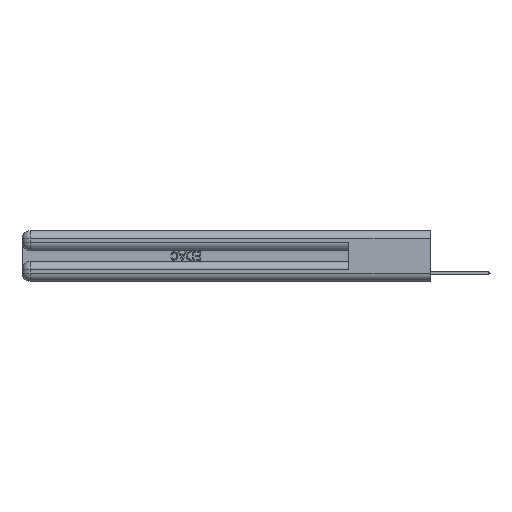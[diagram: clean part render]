
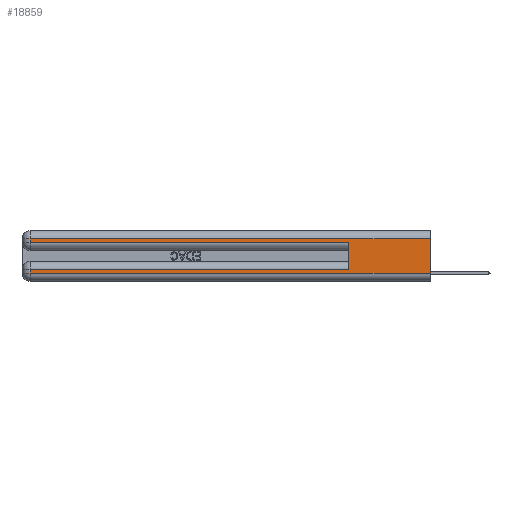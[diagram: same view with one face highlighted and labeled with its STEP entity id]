
A CAD part, left-side view. The second image highlights one B-rep face of the part: STEP entity #18859.
In plain terms, the highlighted planar face has unit normal (-1, 0, 0).
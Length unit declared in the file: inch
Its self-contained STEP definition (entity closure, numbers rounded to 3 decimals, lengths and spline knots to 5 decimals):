
#76 = CARTESIAN_POINT ( 'NONE',  ( 0., 2.94, 0.285 ) ) ;
#77 = DIRECTION ( 'NONE',  ( 0., 1., 0. ) ) ;
#915 = VERTEX_POINT ( 'NONE', #26305 ) ;
#960 = CARTESIAN_POINT ( 'NONE',  ( 0., 2.94, 0.085 ) ) ;
#1370 = DIRECTION ( 'NONE',  ( 0., 1., 0. ) ) ;
#1757 = CARTESIAN_POINT ( 'NONE',  ( 0., 0., 0.085 ) ) ;
#2196 = LINE ( 'NONE', #12408, #24344 ) ;
#2797 = VECTOR ( 'NONE', #77, 39.37008 ) ;
#3200 = VERTEX_POINT ( 'NONE', #20789 ) ;
#4183 = DIRECTION ( 'NONE',  ( 0., 0., -1. ) ) ;
#4246 = LINE ( 'NONE', #13403, #15319 ) ;
#4471 = VECTOR ( 'NONE', #8225, 39.37008 ) ;
#4505 = EDGE_CURVE ( 'NONE', #9222, #26386, #4246, .T. ) ;
#4554 = VECTOR ( 'NONE', #13095, 39.37008 ) ;
#5311 = EDGE_CURVE ( 'NONE', #12001, #16558, #11518, .T. ) ;
#6048 = AXIS2_PLACEMENT_3D ( 'NONE', #17595, #20907, #12003 ) ;
#7359 = ORIENTED_EDGE ( 'NONE', *, *, #26562, .T. ) ;
#8225 = DIRECTION ( 'NONE',  ( 0., 0., -1. ) ) ;
#8251 = CARTESIAN_POINT ( 'NONE',  ( 0., 2.94, 0.37 ) ) ;
#9196 = ORIENTED_EDGE ( 'NONE', *, *, #4505, .F. ) ;
#9222 = VERTEX_POINT ( 'NONE', #20706 ) ;
#9825 = ORIENTED_EDGE ( 'NONE', *, *, #13390, .F. ) ;
#10699 = CARTESIAN_POINT ( 'NONE',  ( 0., 0., 0.285 ) ) ;
#11518 = LINE ( 'NONE', #1757, #2797 ) ;
#12001 = VERTEX_POINT ( 'NONE', #29136 ) ;
#12003 = DIRECTION ( 'NONE',  ( 0., 0., -1. ) ) ;
#12088 = ORIENTED_EDGE ( 'NONE', *, *, #16256, .T. ) ;
#12408 = CARTESIAN_POINT ( 'NONE',  ( 0., 0., 0.06 ) ) ;
#12576 = VERTEX_POINT ( 'NONE', #21124 ) ;
#13095 = DIRECTION ( 'NONE',  ( 0., -1., 0. ) ) ;
#13332 = LINE ( 'NONE', #8251, #26271 ) ;
#13390 = EDGE_CURVE ( 'NONE', #12001, #12576, #27949, .T. ) ;
#13403 = CARTESIAN_POINT ( 'NONE',  ( 0., 0., 0.37 ) ) ;
#14006 = ORIENTED_EDGE ( 'NONE', *, *, #20145, .T. ) ;
#14371 = DIRECTION ( 'NONE',  ( 0., -1., 0. ) ) ;
#14449 = EDGE_CURVE ( 'NONE', #16558, #915, #13332, .T. ) ;
#14635 = EDGE_CURVE ( 'NONE', #915, #26386, #2196, .T. ) ;
#15008 = ORIENTED_EDGE ( 'NONE', *, *, #14635, .T. ) ;
#15319 = VECTOR ( 'NONE', #22906, 39.37008 ) ;
#15427 = CARTESIAN_POINT ( 'NONE',  ( 0., 0., 0.06 ) ) ;
#16256 = EDGE_CURVE ( 'NONE', #3200, #17463, #19938, .T. ) ;
#16558 = VERTEX_POINT ( 'NONE', #960 ) ;
#17441 = ORIENTED_EDGE ( 'NONE', *, *, #5311, .T. ) ;
#17463 = VERTEX_POINT ( 'NONE', #76 ) ;
#17465 = LINE ( 'NONE', #19732, #19450 ) ;
#17595 = CARTESIAN_POINT ( 'NONE',  ( 0., 0., 0.37 ) ) ;
#17645 = LINE ( 'NONE', #10699, #4554 ) ;
#18859 = ADVANCED_FACE ( 'NONE', ( #24674 ), #22419, .F. ) ;
#19450 = VECTOR ( 'NONE', #1370, 39.37008 ) ;
#19626 = VECTOR ( 'NONE', #25542, 39.37008 ) ;
#19732 = CARTESIAN_POINT ( 'NONE',  ( 0., 0., 0.31 ) ) ;
#19938 = LINE ( 'NONE', #29139, #4471 ) ;
#20145 = EDGE_CURVE ( 'NONE', #17463, #12576, #17645, .T. ) ;
#20706 = CARTESIAN_POINT ( 'NONE',  ( 0., 0., 0.31 ) ) ;
#20789 = CARTESIAN_POINT ( 'NONE',  ( 0., 2.94, 0.31 ) ) ;
#20879 = CARTESIAN_POINT ( 'NONE',  ( 0., 0.6, 0.145 ) ) ;
#20907 = DIRECTION ( 'NONE',  ( 1., 0., 0. ) ) ;
#21124 = CARTESIAN_POINT ( 'NONE',  ( 0., 0.6, 0.285 ) ) ;
#22419 = PLANE ( 'NONE',  #6048 ) ;
#22906 = DIRECTION ( 'NONE',  ( 0., 0., -1. ) ) ;
#24344 = VECTOR ( 'NONE', #14371, 39.37008 ) ;
#24674 = FACE_OUTER_BOUND ( 'NONE', #28329, .T. ) ;
#25542 = DIRECTION ( 'NONE',  ( 0., 0., 1. ) ) ;
#25727 = ORIENTED_EDGE ( 'NONE', *, *, #14449, .T. ) ;
#26271 = VECTOR ( 'NONE', #4183, 39.37008 ) ;
#26305 = CARTESIAN_POINT ( 'NONE',  ( 0., 2.94, 0.06 ) ) ;
#26386 = VERTEX_POINT ( 'NONE', #15427 ) ;
#26562 = EDGE_CURVE ( 'NONE', #9222, #3200, #17465, .T. ) ;
#27949 = LINE ( 'NONE', #20879, #19626 ) ;
#28329 = EDGE_LOOP ( 'NONE', ( #9196, #7359, #12088, #14006, #9825, #17441, #25727, #15008 ) ) ;
#29136 = CARTESIAN_POINT ( 'NONE',  ( 0., 0.6, 0.085 ) ) ;
#29139 = CARTESIAN_POINT ( 'NONE',  ( 0., 2.94, 0.37 ) ) ;
